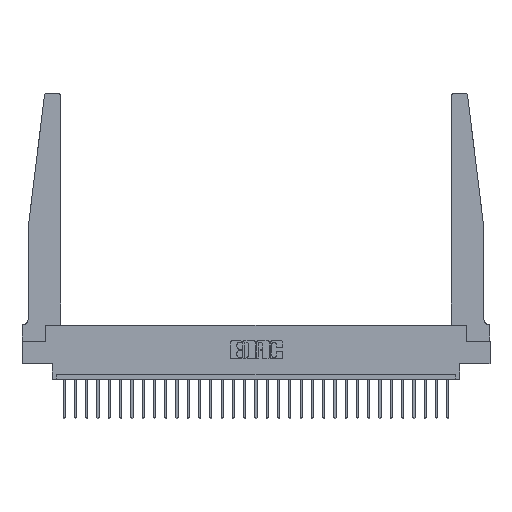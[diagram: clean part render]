
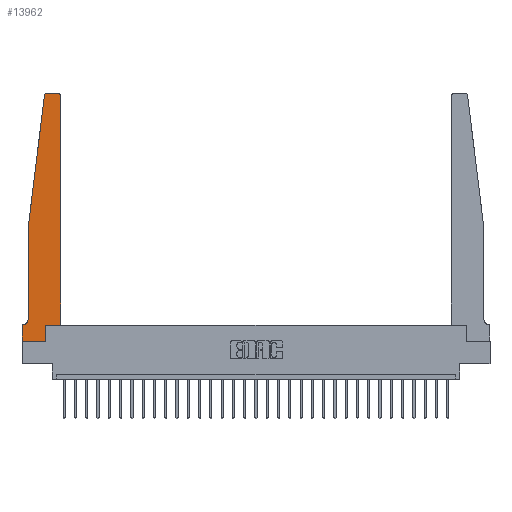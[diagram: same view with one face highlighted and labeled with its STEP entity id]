
A CAD part, top view. The second image highlights one B-rep face of the part: STEP entity #13962.
In plain terms, the highlighted planar face has unit normal (0, 0, 1).
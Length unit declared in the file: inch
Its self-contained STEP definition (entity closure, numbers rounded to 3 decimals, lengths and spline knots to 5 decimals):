
#561 = DIRECTION ( 'NONE',  ( -0.122, -0.992, 0. ) ) ;
#726 = EDGE_CURVE ( 'NONE', #24430, #24981, #9986, .T. ) ;
#754 = DIRECTION ( 'NONE',  ( -1., 0., 0. ) ) ;
#1368 = CARTESIAN_POINT ( 'NONE',  ( 0.425, 0.18, 0.37 ) ) ;
#1371 = EDGE_CURVE ( 'NONE', #24891, #18596, #13289, .T. ) ;
#1651 = ORIENTED_EDGE ( 'NONE', *, *, #1371, .T. ) ;
#2286 = ORIENTED_EDGE ( 'NONE', *, *, #26120, .T. ) ;
#2529 = DIRECTION ( 'NONE',  ( 1., 0., 0. ) ) ;
#3392 = DIRECTION ( 'NONE',  ( 0., 1., 0. ) ) ;
#3529 = PLANE ( 'NONE',  #20288 ) ;
#3738 = VECTOR ( 'NONE', #21286, 39.37008 ) ;
#3817 = EDGE_CURVE ( 'NONE', #4219, #4193, #25787, .T. ) ;
#4193 = VERTEX_POINT ( 'NONE', #8175 ) ;
#4219 = VERTEX_POINT ( 'NONE', #23000 ) ;
#4838 = EDGE_CURVE ( 'NONE', #12763, #24430, #17643, .T. ) ;
#5013 = EDGE_CURVE ( 'NONE', #15708, #13966, #20949, .T. ) ;
#5509 = DIRECTION ( 'NONE',  ( 1., 0., 0. ) ) ;
#5543 = CARTESIAN_POINT ( 'NONE',  ( 0.25, 2.75, 0.37 ) ) ;
#5699 = CARTESIAN_POINT ( 'NONE',  ( 0., 0.1875, 0.37 ) ) ;
#5868 = CARTESIAN_POINT ( 'NONE',  ( 0.2605, 0., 0.37 ) ) ;
#5997 = VECTOR ( 'NONE', #754, 39.37008 ) ;
#6137 = FACE_OUTER_BOUND ( 'NONE', #12296, .T. ) ;
#6199 = CARTESIAN_POINT ( 'NONE',  ( 0.015, 0.2375, 0.37 ) ) ;
#6688 = VERTEX_POINT ( 'NONE', #22238 ) ;
#6759 = CARTESIAN_POINT ( 'NONE',  ( 0., 0., 0.37 ) ) ;
#6970 = VERTEX_POINT ( 'NONE', #12812 ) ;
#7029 = EDGE_CURVE ( 'NONE', #4193, #12763, #9796, .T. ) ;
#7463 = DIRECTION ( 'NONE',  ( 1., 0., 0. ) ) ;
#7503 = DIRECTION ( 'NONE',  ( 0., 1., 0. ) ) ;
#7854 = EDGE_CURVE ( 'NONE', #6970, #4219, #25063, .T. ) ;
#8175 = CARTESIAN_POINT ( 'NONE',  ( 0.065, 1.25, 0.37 ) ) ;
#8247 = DIRECTION ( 'NONE',  ( 0., 0., 1. ) ) ;
#9403 = CARTESIAN_POINT ( 'NONE',  ( 0., 0., 0.37 ) ) ;
#9559 = ORIENTED_EDGE ( 'NONE', *, *, #19506, .T. ) ;
#9796 = LINE ( 'NONE', #13173, #17858 ) ;
#9986 = LINE ( 'NONE', #19758, #5997 ) ;
#10420 = LINE ( 'NONE', #11492, #20772 ) ;
#10544 = ORIENTED_EDGE ( 'NONE', *, *, #726, .T. ) ;
#11037 = ORIENTED_EDGE ( 'NONE', *, *, #17198, .T. ) ;
#11109 = ORIENTED_EDGE ( 'NONE', *, *, #12039, .T. ) ;
#11323 = ORIENTED_EDGE ( 'NONE', *, *, #7029, .T. ) ;
#11404 = VERTEX_POINT ( 'NONE', #22163 ) ;
#11492 = CARTESIAN_POINT ( 'NONE',  ( 0.2605, 0.18, 0.37 ) ) ;
#11559 = LINE ( 'NONE', #1368, #23546 ) ;
#11612 = LINE ( 'NONE', #21063, #12633 ) ;
#12039 = EDGE_CURVE ( 'NONE', #6688, #24891, #11559, .T. ) ;
#12296 = EDGE_LOOP ( 'NONE', ( #9559, #13249, #26359, #11323, #18061, #10544, #11037, #15740, #15578, #2286, #11109, #1651 ) ) ;
#12633 = VECTOR ( 'NONE', #23165, 39.37008 ) ;
#12763 = VERTEX_POINT ( 'NONE', #22443 ) ;
#12812 = CARTESIAN_POINT ( 'NONE',  ( 0.27653, 2.75, 0.37 ) ) ;
#12814 = DIRECTION ( 'NONE',  ( 0., 0., -1. ) ) ;
#12999 = CARTESIAN_POINT ( 'NONE',  ( 0., 0.1875, 0.37 ) ) ;
#13063 = CARTESIAN_POINT ( 'NONE',  ( 0.065, 1.25, 0.37 ) ) ;
#13173 = CARTESIAN_POINT ( 'NONE',  ( 0.065, 1.25, 0.37 ) ) ;
#13249 = ORIENTED_EDGE ( 'NONE', *, *, #7854, .T. ) ;
#13289 = CIRCLE ( 'NONE', #19901, 0.03 ) ;
#13962 = ADVANCED_FACE ( 'NONE', ( #6137 ), #3529, .T. ) ;
#13966 = VERTEX_POINT ( 'NONE', #5868 ) ;
#14106 = CARTESIAN_POINT ( 'NONE',  ( 0.27653, 2.72, 0.37 ) ) ;
#14902 = CARTESIAN_POINT ( 'NONE',  ( 0.425, 2.72, 0.37 ) ) ;
#15376 = DIRECTION ( 'NONE',  ( 0., -1., 0. ) ) ;
#15578 = ORIENTED_EDGE ( 'NONE', *, *, #16837, .T. ) ;
#15708 = VERTEX_POINT ( 'NONE', #9403 ) ;
#15740 = ORIENTED_EDGE ( 'NONE', *, *, #5013, .T. ) ;
#16837 = EDGE_CURVE ( 'NONE', #13966, #11404, #10420, .T. ) ;
#17198 = EDGE_CURVE ( 'NONE', #24981, #15708, #25356, .T. ) ;
#17326 = CARTESIAN_POINT ( 'NONE',  ( 0.015, 0.1875, 0.37 ) ) ;
#17643 = CIRCLE ( 'NONE', #25615, 0.05 ) ;
#17858 = VECTOR ( 'NONE', #15376, 39.37008 ) ;
#18058 = DIRECTION ( 'NONE',  ( -1., 0., 0. ) ) ;
#18061 = ORIENTED_EDGE ( 'NONE', *, *, #4838, .T. ) ;
#18297 = DIRECTION ( 'NONE',  ( 0., 0., 1. ) ) ;
#18541 = CARTESIAN_POINT ( 'NONE',  ( 0.395, 2.72, 0.37 ) ) ;
#18596 = VERTEX_POINT ( 'NONE', #18607 ) ;
#18607 = CARTESIAN_POINT ( 'NONE',  ( 0.395, 2.75, 0.37 ) ) ;
#19210 = CARTESIAN_POINT ( 'NONE',  ( 0., 0., 0.37 ) ) ;
#19506 = EDGE_CURVE ( 'NONE', #18596, #6970, #20614, .T. ) ;
#19758 = CARTESIAN_POINT ( 'NONE',  ( 0.065, 0.1875, 0.37 ) ) ;
#19901 = AXIS2_PLACEMENT_3D ( 'NONE', #18541, #8247, #26968 ) ;
#20288 = AXIS2_PLACEMENT_3D ( 'NONE', #5699, #18297, #5509 ) ;
#20614 = LINE ( 'NONE', #5543, #23901 ) ;
#20772 = VECTOR ( 'NONE', #7503, 39.37008 ) ;
#20894 = AXIS2_PLACEMENT_3D ( 'NONE', #14106, #24453, #7463 ) ;
#20949 = LINE ( 'NONE', #6759, #22596 ) ;
#21063 = CARTESIAN_POINT ( 'NONE',  ( 0.425, 0.18, 0.37 ) ) ;
#21286 = DIRECTION ( 'NONE',  ( 0., -1., 0. ) ) ;
#22163 = CARTESIAN_POINT ( 'NONE',  ( 0.2605, 0.18, 0.37 ) ) ;
#22238 = CARTESIAN_POINT ( 'NONE',  ( 0.425, 0.18, 0.37 ) ) ;
#22443 = CARTESIAN_POINT ( 'NONE',  ( 0.065, 0.2375, 0.37 ) ) ;
#22596 = VECTOR ( 'NONE', #2529, 39.37008 ) ;
#23000 = CARTESIAN_POINT ( 'NONE',  ( 0.24675, 2.72367, 0.37 ) ) ;
#23165 = DIRECTION ( 'NONE',  ( 1., 0., 0. ) ) ;
#23237 = DIRECTION ( 'NONE',  ( -1., 0., 0. ) ) ;
#23546 = VECTOR ( 'NONE', #3392, 39.37008 ) ;
#23901 = VECTOR ( 'NONE', #18058, 39.37008 ) ;
#24430 = VERTEX_POINT ( 'NONE', #17326 ) ;
#24453 = DIRECTION ( 'NONE',  ( 0., 0., 1. ) ) ;
#24891 = VERTEX_POINT ( 'NONE', #14902 ) ;
#24981 = VERTEX_POINT ( 'NONE', #12999 ) ;
#25063 = CIRCLE ( 'NONE', #20894, 0.03 ) ;
#25356 = LINE ( 'NONE', #19210, #3738 ) ;
#25615 = AXIS2_PLACEMENT_3D ( 'NONE', #6199, #12814, #23237 ) ;
#25787 = LINE ( 'NONE', #13063, #25964 ) ;
#25964 = VECTOR ( 'NONE', #561, 39.37008 ) ;
#26120 = EDGE_CURVE ( 'NONE', #11404, #6688, #11612, .T. ) ;
#26359 = ORIENTED_EDGE ( 'NONE', *, *, #3817, .T. ) ;
#26968 = DIRECTION ( 'NONE',  ( 1., 0., 0. ) ) ;
